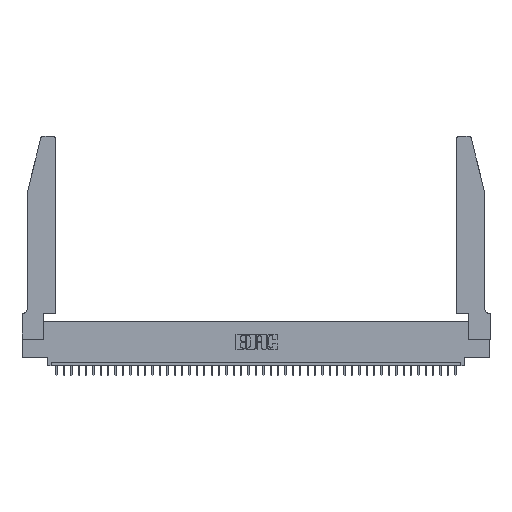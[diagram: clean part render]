
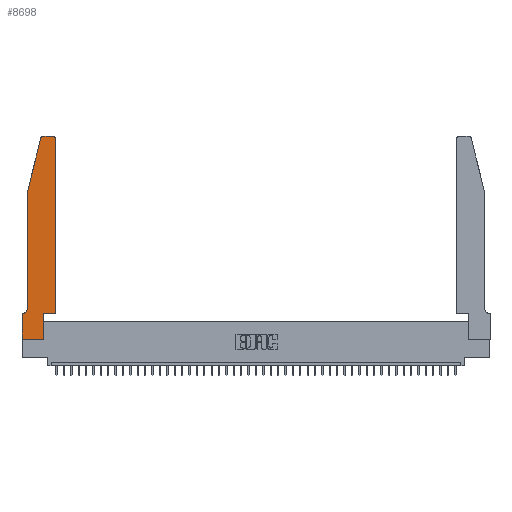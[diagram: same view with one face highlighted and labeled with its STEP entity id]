
A CAD part, top view. The second image highlights one B-rep face of the part: STEP entity #8698.
In plain terms, the highlighted planar face has unit normal (0, 0, 1).
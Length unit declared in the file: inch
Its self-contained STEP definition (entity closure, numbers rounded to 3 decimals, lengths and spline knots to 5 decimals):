
#924 = CARTESIAN_POINT ( 'NONE',  ( 0.0055, 0.35, 0.37 ) ) ;
#2018 = LINE ( 'NONE', #30008, #26667 ) ;
#2053 = VERTEX_POINT ( 'NONE', #24388 ) ;
#2277 = CARTESIAN_POINT ( 'NONE',  ( 0.2605, 2.75, 0.37 ) ) ;
#2328 = CARTESIAN_POINT ( 'NONE',  ( 0., 0., 0.37 ) ) ;
#2530 = EDGE_CURVE ( 'NONE', #33114, #12030, #8298, .T. ) ;
#2644 = LINE ( 'NONE', #43490, #6051 ) ;
#3193 = VECTOR ( 'NONE', #43819, 39.37008 ) ;
#3688 = VECTOR ( 'NONE', #42826, 39.37008 ) ;
#3798 = CARTESIAN_POINT ( 'NONE',  ( 0.2865, 0., 0.37 ) ) ;
#3892 = CARTESIAN_POINT ( 'NONE',  ( 0.2865, 0.35, 0.37 ) ) ;
#4139 = VECTOR ( 'NONE', #14918, 39.37008 ) ;
#6051 = VECTOR ( 'NONE', #8732, 39.37008 ) ;
#6286 = VERTEX_POINT ( 'NONE', #15167 ) ;
#6514 = ORIENTED_EDGE ( 'NONE', *, *, #18048, .T. ) ;
#7694 = FACE_OUTER_BOUND ( 'NONE', #14790, .T. ) ;
#7915 = DIRECTION ( 'NONE',  ( 1., 0., 0. ) ) ;
#8132 = CARTESIAN_POINT ( 'NONE',  ( 0., 0.35, 0.37 ) ) ;
#8136 = VERTEX_POINT ( 'NONE', #10693 ) ;
#8298 = LINE ( 'NONE', #39228, #3688 ) ;
#8698 = ADVANCED_FACE ( 'NONE', ( #7694 ), #21456, .T. ) ;
#8732 = DIRECTION ( 'NONE',  ( 0., -1., 0. ) ) ;
#9290 = CARTESIAN_POINT ( 'NONE',  ( 0.284, 2.72, 0.37 ) ) ;
#10693 = CARTESIAN_POINT ( 'NONE',  ( 0.0755, 0.42, 0.37 ) ) ;
#11072 = CARTESIAN_POINT ( 'NONE',  ( 0., 0., 0.37 ) ) ;
#11785 = EDGE_CURVE ( 'NONE', #6286, #33114, #21885, .T. ) ;
#12010 = ORIENTED_EDGE ( 'NONE', *, *, #19218, .T. ) ;
#12030 = VERTEX_POINT ( 'NONE', #3798 ) ;
#12257 = CARTESIAN_POINT ( 'NONE',  ( 0.2865, 0.35, 0.37 ) ) ;
#12954 = AXIS2_PLACEMENT_3D ( 'NONE', #30068, #39551, #43603 ) ;
#14223 = VERTEX_POINT ( 'NONE', #40499 ) ;
#14397 = ORIENTED_EDGE ( 'NONE', *, *, #41676, .T. ) ;
#14705 = ORIENTED_EDGE ( 'NONE', *, *, #33119, .T. ) ;
#14722 = VECTOR ( 'NONE', #28725, 39.37008 ) ;
#14790 = EDGE_LOOP ( 'NONE', ( #20815, #12010, #35610, #39440, #32399, #14397, #27077, #20073, #14705, #6514, #17749, #17247 ) ) ;
#14918 = DIRECTION ( 'NONE',  ( 0., -1., 0. ) ) ;
#14953 = VERTEX_POINT ( 'NONE', #16250 ) ;
#15167 = CARTESIAN_POINT ( 'NONE',  ( 0., 0.35, 0.37 ) ) ;
#15217 = AXIS2_PLACEMENT_3D ( 'NONE', #9290, #18764, #39550 ) ;
#15583 = VECTOR ( 'NONE', #16039, 39.37008 ) ;
#16039 = DIRECTION ( 'NONE',  ( -1., 0., 0. ) ) ;
#16250 = CARTESIAN_POINT ( 'NONE',  ( 0.4505, 2.72, 0.37 ) ) ;
#16284 = LINE ( 'NONE', #40207, #3193 ) ;
#16548 = DIRECTION ( 'NONE',  ( 0., 0., -1. ) ) ;
#17061 = AXIS2_PLACEMENT_3D ( 'NONE', #26699, #16548, #23308 ) ;
#17247 = ORIENTED_EDGE ( 'NONE', *, *, #17687, .T. ) ;
#17687 = EDGE_CURVE ( 'NONE', #14953, #14223, #27376, .T. ) ;
#17749 = ORIENTED_EDGE ( 'NONE', *, *, #41785, .T. ) ;
#18048 = EDGE_CURVE ( 'NONE', #26924, #42289, #2018, .T. ) ;
#18585 = LINE ( 'NONE', #12257, #41248 ) ;
#18764 = DIRECTION ( 'NONE',  ( 0., 0., 1. ) ) ;
#18913 = DIRECTION ( 'NONE',  ( -0.239, -0.971, 0. ) ) ;
#19218 = EDGE_CURVE ( 'NONE', #35517, #27693, #42618, .T. ) ;
#20073 = ORIENTED_EDGE ( 'NONE', *, *, #2530, .T. ) ;
#20815 = ORIENTED_EDGE ( 'NONE', *, *, #38791, .T. ) ;
#21456 = PLANE ( 'NONE',  #37791 ) ;
#21487 = CARTESIAN_POINT ( 'NONE',  ( 0.0755, 0.35, 0.37 ) ) ;
#21682 = DIRECTION ( 'NONE',  ( 0., 0., 1. ) ) ;
#21885 = LINE ( 'NONE', #11072, #4139 ) ;
#23308 = DIRECTION ( 'NONE',  ( -1., 0., 0. ) ) ;
#24005 = VERTEX_POINT ( 'NONE', #924 ) ;
#24029 = LINE ( 'NONE', #21487, #14722 ) ;
#24388 = CARTESIAN_POINT ( 'NONE',  ( 0.0755, 2., 0.37 ) ) ;
#26667 = VECTOR ( 'NONE', #39278, 39.37008 ) ;
#26699 = CARTESIAN_POINT ( 'NONE',  ( 0.0055, 0.42, 0.37 ) ) ;
#26924 = VERTEX_POINT ( 'NONE', #3892 ) ;
#27077 = ORIENTED_EDGE ( 'NONE', *, *, #11785, .T. ) ;
#27173 = CIRCLE ( 'NONE', #17061, 0.07 ) ;
#27376 = CIRCLE ( 'NONE', #12954, 0.03 ) ;
#27465 = EDGE_CURVE ( 'NONE', #8136, #24005, #27173, .T. ) ;
#27693 = VERTEX_POINT ( 'NONE', #36300 ) ;
#27703 = EDGE_CURVE ( 'NONE', #27693, #2053, #36084, .T. ) ;
#28725 = DIRECTION ( 'NONE',  ( -1., 0., 0. ) ) ;
#30008 = CARTESIAN_POINT ( 'NONE',  ( 0.4505, 0.35, 0.37 ) ) ;
#30068 = CARTESIAN_POINT ( 'NONE',  ( 0.4205, 2.72, 0.37 ) ) ;
#32288 = CARTESIAN_POINT ( 'NONE',  ( 0.284, 2.75, 0.37 ) ) ;
#32399 = ORIENTED_EDGE ( 'NONE', *, *, #27465, .T. ) ;
#32584 = DIRECTION ( 'NONE',  ( 0., 1., 0. ) ) ;
#32934 = CARTESIAN_POINT ( 'NONE',  ( 0.0755, 2., 0.37 ) ) ;
#33114 = VERTEX_POINT ( 'NONE', #2328 ) ;
#33119 = EDGE_CURVE ( 'NONE', #12030, #26924, #18585, .T. ) ;
#33652 = LINE ( 'NONE', #2277, #15583 ) ;
#35517 = VERTEX_POINT ( 'NONE', #32288 ) ;
#35610 = ORIENTED_EDGE ( 'NONE', *, *, #27703, .T. ) ;
#36084 = LINE ( 'NONE', #32934, #36531 ) ;
#36300 = CARTESIAN_POINT ( 'NONE',  ( 0.25487, 2.72718, 0.37 ) ) ;
#36304 = CARTESIAN_POINT ( 'NONE',  ( 0.4505, 0.35, 0.37 ) ) ;
#36531 = VECTOR ( 'NONE', #18913, 39.37008 ) ;
#37791 = AXIS2_PLACEMENT_3D ( 'NONE', #8132, #21682, #7915 ) ;
#38791 = EDGE_CURVE ( 'NONE', #14223, #35517, #33652, .T. ) ;
#39228 = CARTESIAN_POINT ( 'NONE',  ( 0., 0., 0.37 ) ) ;
#39278 = DIRECTION ( 'NONE',  ( 1., 0., 0. ) ) ;
#39440 = ORIENTED_EDGE ( 'NONE', *, *, #43508, .T. ) ;
#39550 = DIRECTION ( 'NONE',  ( 1., 0., 0. ) ) ;
#39551 = DIRECTION ( 'NONE',  ( 0., 0., 1. ) ) ;
#40207 = CARTESIAN_POINT ( 'NONE',  ( 0.4505, 0.35, 0.37 ) ) ;
#40499 = CARTESIAN_POINT ( 'NONE',  ( 0.4205, 2.75, 0.37 ) ) ;
#41248 = VECTOR ( 'NONE', #32584, 39.37008 ) ;
#41676 = EDGE_CURVE ( 'NONE', #24005, #6286, #24029, .T. ) ;
#41785 = EDGE_CURVE ( 'NONE', #42289, #14953, #16284, .T. ) ;
#42289 = VERTEX_POINT ( 'NONE', #36304 ) ;
#42618 = CIRCLE ( 'NONE', #15217, 0.03 ) ;
#42826 = DIRECTION ( 'NONE',  ( 1., 0., 0. ) ) ;
#43490 = CARTESIAN_POINT ( 'NONE',  ( 0.0755, 2., 0.37 ) ) ;
#43508 = EDGE_CURVE ( 'NONE', #2053, #8136, #2644, .T. ) ;
#43603 = DIRECTION ( 'NONE',  ( 1., 0., 0. ) ) ;
#43819 = DIRECTION ( 'NONE',  ( 0., 1., 0. ) ) ;
